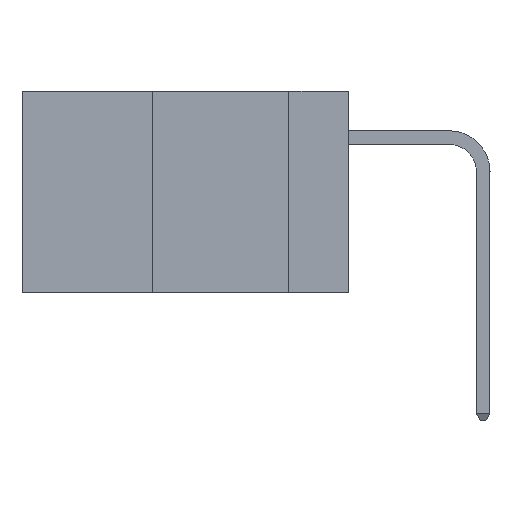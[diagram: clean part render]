
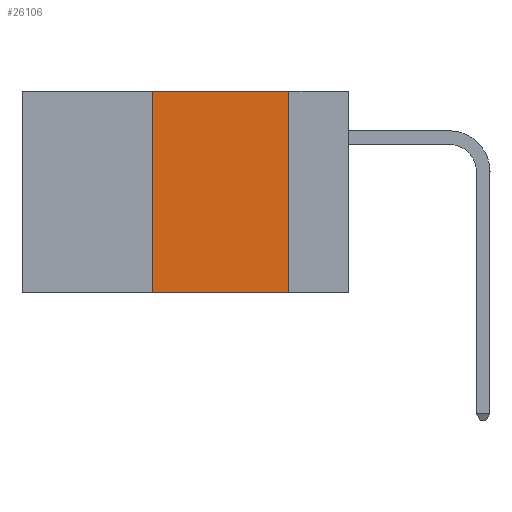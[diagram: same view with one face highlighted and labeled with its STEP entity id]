
A CAD part, left-side view. The second image highlights one B-rep face of the part: STEP entity #26106.
In plain terms, the highlighted planar face has unit normal (-1, 0, 0).
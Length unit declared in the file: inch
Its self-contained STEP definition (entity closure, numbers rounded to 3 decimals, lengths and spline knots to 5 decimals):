
#45 = LINE ( 'NONE', #27580, #38267 ) ;
#683 = VECTOR ( 'NONE', #21865, 39.37008 ) ;
#737 = CARTESIAN_POINT ( 'NONE',  ( 0., 0.11, -0.37 ) ) ;
#2491 = DIRECTION ( 'NONE',  ( 0., -1., 0. ) ) ;
#3453 = CARTESIAN_POINT ( 'NONE',  ( 0., 0.6, 0. ) ) ;
#3709 = CARTESIAN_POINT ( 'NONE',  ( 0., 0.6, -0.37 ) ) ;
#4027 = VECTOR ( 'NONE', #16009, 39.37008 ) ;
#5626 = CARTESIAN_POINT ( 'NONE',  ( 0., 0.6, 0. ) ) ;
#5708 = CARTESIAN_POINT ( 'NONE',  ( 0., 0.11, 0. ) ) ;
#5970 = AXIS2_PLACEMENT_3D ( 'NONE', #3453, #6576, #27597 ) ;
#6576 = DIRECTION ( 'NONE',  ( 1., 0., 0. ) ) ;
#6999 = LINE ( 'NONE', #15890, #683 ) ;
#7415 = VERTEX_POINT ( 'NONE', #737 ) ;
#12839 = VERTEX_POINT ( 'NONE', #5708 ) ;
#14498 = VERTEX_POINT ( 'NONE', #25859 ) ;
#15752 = DIRECTION ( 'NONE',  ( 0., 0., 1. ) ) ;
#15890 = CARTESIAN_POINT ( 'NONE',  ( 0., 0.11, 0. ) ) ;
#16009 = DIRECTION ( 'NONE',  ( 0., -1., 0. ) ) ;
#18544 = VECTOR ( 'NONE', #2491, 39.37008 ) ;
#20873 = ORIENTED_EDGE ( 'NONE', *, *, #22289, .T. ) ;
#21618 = PLANE ( 'NONE',  #5970 ) ;
#21865 = DIRECTION ( 'NONE',  ( 0., 0., -1. ) ) ;
#22289 = EDGE_CURVE ( 'NONE', #27350, #7415, #29034, .T. ) ;
#23297 = FACE_OUTER_BOUND ( 'NONE', #25099, .T. ) ;
#25099 = EDGE_LOOP ( 'NONE', ( #25961, #34908, #35852, #20873 ) ) ;
#25859 = CARTESIAN_POINT ( 'NONE',  ( 0., 0.36, 0. ) ) ;
#25961 = ORIENTED_EDGE ( 'NONE', *, *, #30227, .F. ) ;
#26106 = ADVANCED_FACE ( 'NONE', ( #23297 ), #21618, .F. ) ;
#27133 = EDGE_CURVE ( 'NONE', #14498, #12839, #34454, .T. ) ;
#27350 = VERTEX_POINT ( 'NONE', #37131 ) ;
#27580 = CARTESIAN_POINT ( 'NONE',  ( 0., 0.36, 0. ) ) ;
#27597 = DIRECTION ( 'NONE',  ( 0., 0., -1. ) ) ;
#29034 = LINE ( 'NONE', #3709, #4027 ) ;
#30227 = EDGE_CURVE ( 'NONE', #12839, #7415, #6999, .T. ) ;
#33275 = EDGE_CURVE ( 'NONE', #27350, #14498, #45, .T. ) ;
#34454 = LINE ( 'NONE', #5626, #18544 ) ;
#34908 = ORIENTED_EDGE ( 'NONE', *, *, #27133, .F. ) ;
#35852 = ORIENTED_EDGE ( 'NONE', *, *, #33275, .F. ) ;
#37131 = CARTESIAN_POINT ( 'NONE',  ( 0., 0.36, -0.37 ) ) ;
#38267 = VECTOR ( 'NONE', #15752, 39.37008 ) ;
